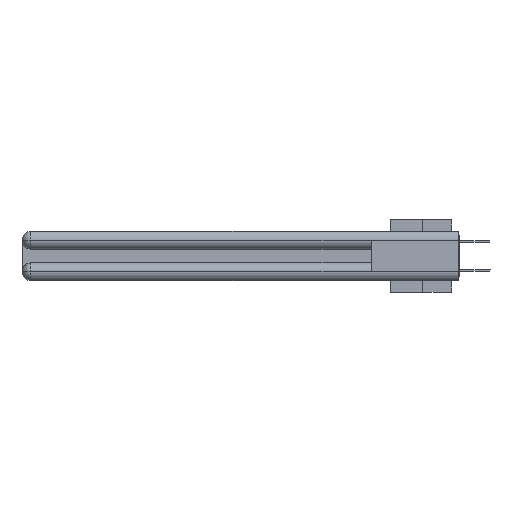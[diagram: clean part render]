
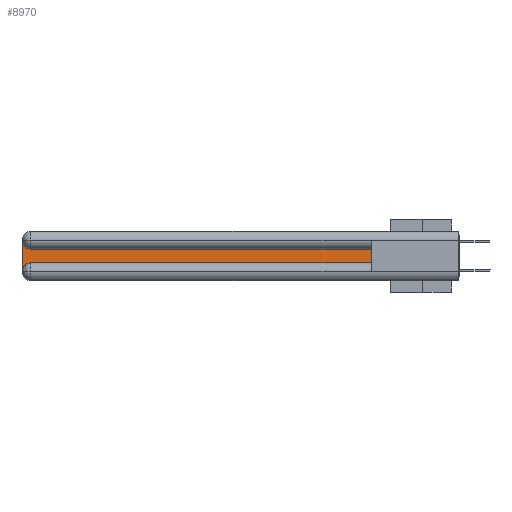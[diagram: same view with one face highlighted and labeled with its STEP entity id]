
A CAD part, left-side view. The second image highlights one B-rep face of the part: STEP entity #8970.
In plain terms, the highlighted planar face has unit normal (-1, 0, 0).
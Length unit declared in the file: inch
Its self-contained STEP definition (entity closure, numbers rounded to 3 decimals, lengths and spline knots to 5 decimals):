
#862 = AXIS2_PLACEMENT_3D ( 'NONE', #28868, #4821, #21666 ) ;
#1795 = AXIS2_PLACEMENT_3D ( 'NONE', #1989, #11841, #16709 ) ;
#1989 = CARTESIAN_POINT ( 'NONE',  ( 0.075, 2.94, -0.0625 ) ) ;
#1998 = VERTEX_POINT ( 'NONE', #19407 ) ;
#2480 = CARTESIAN_POINT ( 'NONE',  ( 0.075, 3., -0.2775 ) ) ;
#2680 = DIRECTION ( 'NONE',  ( 0., 0., 1. ) ) ;
#2727 = EDGE_CURVE ( 'NONE', #26981, #18038, #26046, .T. ) ;
#4218 = VECTOR ( 'NONE', #5773, 39.37008 ) ;
#4821 = DIRECTION ( 'NONE',  ( 1., 0., 0. ) ) ;
#5557 = CARTESIAN_POINT ( 'NONE',  ( 0.075, 0.6, -0.1225 ) ) ;
#5773 = DIRECTION ( 'NONE',  ( 0., 0., -1. ) ) ;
#6219 = LINE ( 'NONE', #12316, #14149 ) ;
#7322 = EDGE_CURVE ( 'NONE', #9193, #8484, #19012, .T. ) ;
#7511 = DIRECTION ( 'NONE',  ( 0., -1., 0. ) ) ;
#7592 = LINE ( 'NONE', #29181, #22342 ) ;
#7896 = CIRCLE ( 'NONE', #1795, 0.06 ) ;
#8484 = VERTEX_POINT ( 'NONE', #2480 ) ;
#8970 = ADVANCED_FACE ( 'NONE', ( #27694 ), #11595, .F. ) ;
#9158 = ORIENTED_EDGE ( 'NONE', *, *, #7322, .T. ) ;
#9193 = VERTEX_POINT ( 'NONE', #18246 ) ;
#11595 = PLANE ( 'NONE',  #862 ) ;
#11841 = DIRECTION ( 'NONE',  ( 1., 0., 0. ) ) ;
#11985 = ORIENTED_EDGE ( 'NONE', *, *, #24049, .T. ) ;
#12316 = CARTESIAN_POINT ( 'NONE',  ( 0.075, 0.6, -0.2175 ) ) ;
#12612 = CARTESIAN_POINT ( 'NONE',  ( 0.075, 0.6, -0.2175 ) ) ;
#14149 = VECTOR ( 'NONE', #2680, 39.37008 ) ;
#15453 = DIRECTION ( 'NONE',  ( 1., 0., 0. ) ) ;
#16221 = CARTESIAN_POINT ( 'NONE',  ( 0.075, 2.94, -0.2175 ) ) ;
#16709 = DIRECTION ( 'NONE',  ( 0., 0., -1. ) ) ;
#18038 = VERTEX_POINT ( 'NONE', #12612 ) ;
#18246 = CARTESIAN_POINT ( 'NONE',  ( 0.075, 3., -0.0625 ) ) ;
#19012 = LINE ( 'NONE', #19637, #4218 ) ;
#19013 = DIRECTION ( 'NONE',  ( 0., 1., 0. ) ) ;
#19407 = CARTESIAN_POINT ( 'NONE',  ( 0.075, 2.94, -0.1225 ) ) ;
#19637 = CARTESIAN_POINT ( 'NONE',  ( 0.075, 3., -0.2175 ) ) ;
#20911 = EDGE_CURVE ( 'NONE', #18038, #29672, #6219, .T. ) ;
#21012 = ORIENTED_EDGE ( 'NONE', *, *, #2727, .T. ) ;
#21582 = EDGE_CURVE ( 'NONE', #8484, #26981, #24366, .T. ) ;
#21666 = DIRECTION ( 'NONE',  ( 0., 0., -1. ) ) ;
#22342 = VECTOR ( 'NONE', #19013, 39.37008 ) ;
#22908 = CARTESIAN_POINT ( 'NONE',  ( 0.075, 2.94, -0.2775 ) ) ;
#24049 = EDGE_CURVE ( 'NONE', #29672, #1998, #7592, .T. ) ;
#24125 = VECTOR ( 'NONE', #7511, 39.37008 ) ;
#24366 = CIRCLE ( 'NONE', #24904, 0.06 ) ;
#24904 = AXIS2_PLACEMENT_3D ( 'NONE', #22908, #15453, #27743 ) ;
#25250 = EDGE_CURVE ( 'NONE', #1998, #9193, #7896, .T. ) ;
#26046 = LINE ( 'NONE', #27715, #24125 ) ;
#26915 = ORIENTED_EDGE ( 'NONE', *, *, #25250, .T. ) ;
#26981 = VERTEX_POINT ( 'NONE', #16221 ) ;
#27369 = ORIENTED_EDGE ( 'NONE', *, *, #21582, .T. ) ;
#27694 = FACE_OUTER_BOUND ( 'NONE', #27712, .T. ) ;
#27712 = EDGE_LOOP ( 'NONE', ( #11985, #26915, #9158, #27369, #21012, #31387 ) ) ;
#27715 = CARTESIAN_POINT ( 'NONE',  ( 0.075, 0.6, -0.2175 ) ) ;
#27743 = DIRECTION ( 'NONE',  ( 0., 0., -1. ) ) ;
#28868 = CARTESIAN_POINT ( 'NONE',  ( 0.075, 3., -0.1225 ) ) ;
#29181 = CARTESIAN_POINT ( 'NONE',  ( 0.075, 0.6, -0.1225 ) ) ;
#29672 = VERTEX_POINT ( 'NONE', #5557 ) ;
#31387 = ORIENTED_EDGE ( 'NONE', *, *, #20911, .T. ) ;
